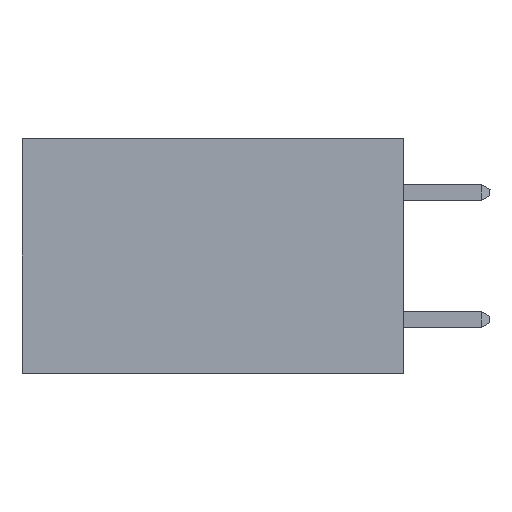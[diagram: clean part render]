
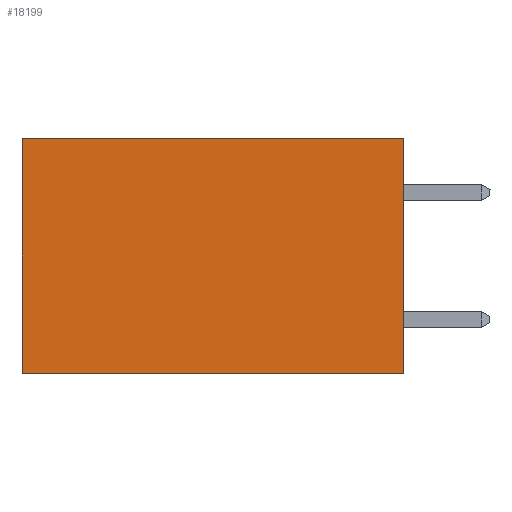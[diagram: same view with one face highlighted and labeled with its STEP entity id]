
A CAD part, left-side view. The second image highlights one B-rep face of the part: STEP entity #18199.
In plain terms, the highlighted planar face has unit normal (-1, 0, 0).
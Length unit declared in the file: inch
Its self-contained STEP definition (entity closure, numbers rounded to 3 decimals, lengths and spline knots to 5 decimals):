
#2975 = VECTOR ( 'NONE', #10220, 39.37008 ) ;
#3908 = PLANE ( 'NONE',  #14195 ) ;
#4176 = CARTESIAN_POINT ( 'NONE',  ( 0.2875, 0., -0.37 ) ) ;
#6625 = VECTOR ( 'NONE', #10639, 39.37008 ) ;
#6679 = DIRECTION ( 'NONE',  ( 0., 0., -1. ) ) ;
#7289 = LINE ( 'NONE', #14673, #6625 ) ;
#8689 = ORIENTED_EDGE ( 'NONE', *, *, #11587, .T. ) ;
#9035 = ORIENTED_EDGE ( 'NONE', *, *, #9731, .F. ) ;
#9731 = EDGE_CURVE ( 'NONE', #23932, #17282, #19642, .T. ) ;
#10202 = DIRECTION ( 'NONE',  ( 0., 0., -1. ) ) ;
#10220 = DIRECTION ( 'NONE',  ( 0., 0., -1. ) ) ;
#10466 = EDGE_CURVE ( 'NONE', #21552, #20942, #7289, .T. ) ;
#10583 = ORIENTED_EDGE ( 'NONE', *, *, #10466, .T. ) ;
#10639 = DIRECTION ( 'NONE',  ( 0., 1., 0. ) ) ;
#11173 = EDGE_LOOP ( 'NONE', ( #8689, #9035, #18926, #10583 ) ) ;
#11587 = EDGE_CURVE ( 'NONE', #20942, #17282, #23886, .T. ) ;
#11965 = CARTESIAN_POINT ( 'NONE',  ( 0.2875, 0.6, 0. ) ) ;
#13716 = VECTOR ( 'NONE', #22417, 39.37008 ) ;
#14195 = AXIS2_PLACEMENT_3D ( 'NONE', #16085, #22161, #10202 ) ;
#14574 = LINE ( 'NONE', #20807, #24545 ) ;
#14673 = CARTESIAN_POINT ( 'NONE',  ( 0.2875, 0., 0. ) ) ;
#15371 = FACE_OUTER_BOUND ( 'NONE', #11173, .T. ) ;
#15991 = CARTESIAN_POINT ( 'NONE',  ( 0.2875, 0., 0. ) ) ;
#16085 = CARTESIAN_POINT ( 'NONE',  ( 0.2875, 0., 0. ) ) ;
#17282 = VERTEX_POINT ( 'NONE', #19275 ) ;
#18199 = ADVANCED_FACE ( 'NONE', ( #15371 ), #3908, .F. ) ;
#18926 = ORIENTED_EDGE ( 'NONE', *, *, #24623, .F. ) ;
#19275 = CARTESIAN_POINT ( 'NONE',  ( 0.2875, 0.6, -0.37 ) ) ;
#19642 = LINE ( 'NONE', #4176, #13716 ) ;
#20192 = CARTESIAN_POINT ( 'NONE',  ( 0.2875, 0.6, 0. ) ) ;
#20752 = CARTESIAN_POINT ( 'NONE',  ( 0.2875, 0., -0.37 ) ) ;
#20807 = CARTESIAN_POINT ( 'NONE',  ( 0.2875, 0., 0. ) ) ;
#20942 = VERTEX_POINT ( 'NONE', #11965 ) ;
#21552 = VERTEX_POINT ( 'NONE', #15991 ) ;
#22161 = DIRECTION ( 'NONE',  ( 1., 0., 0. ) ) ;
#22417 = DIRECTION ( 'NONE',  ( 0., 1., 0. ) ) ;
#23886 = LINE ( 'NONE', #20192, #2975 ) ;
#23932 = VERTEX_POINT ( 'NONE', #20752 ) ;
#24545 = VECTOR ( 'NONE', #6679, 39.37008 ) ;
#24623 = EDGE_CURVE ( 'NONE', #21552, #23932, #14574, .T. ) ;
